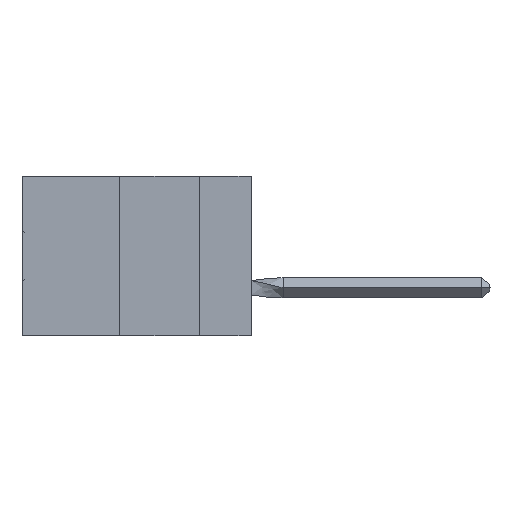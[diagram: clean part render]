
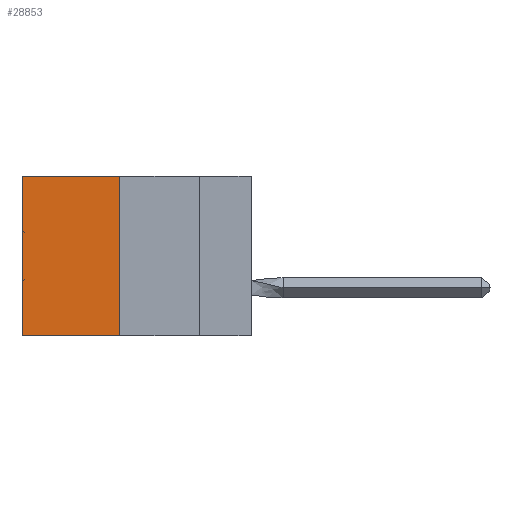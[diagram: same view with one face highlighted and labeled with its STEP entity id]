
A CAD part, left-side view. The second image highlights one B-rep face of the part: STEP entity #28853.
In plain terms, the highlighted planar face has unit normal (-1, 0, 0).
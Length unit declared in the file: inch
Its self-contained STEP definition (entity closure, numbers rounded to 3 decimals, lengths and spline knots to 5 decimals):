
#2161 = CARTESIAN_POINT ( 'NONE',  ( 0.305, 0.413, 0. ) ) ;
#4293 = DIRECTION ( 'NONE',  ( 0., 0., -1. ) ) ;
#4433 = EDGE_LOOP ( 'NONE', ( #32694, #45407, #19764, #10352 ) ) ;
#4659 = CARTESIAN_POINT ( 'NONE',  ( 0.305, 0.72, -0.5 ) ) ;
#6566 = CARTESIAN_POINT ( 'NONE',  ( 0.305, 0.72, -0.5 ) ) ;
#8928 = DIRECTION ( 'NONE',  ( 0., 1., 0. ) ) ;
#9058 = CARTESIAN_POINT ( 'NONE',  ( 0.305, 0.72, 0. ) ) ;
#9150 = EDGE_CURVE ( 'NONE', #37162, #15624, #11273, .T. ) ;
#10037 = DIRECTION ( 'NONE',  ( 0., 1., 0. ) ) ;
#10352 = ORIENTED_EDGE ( 'NONE', *, *, #23976, .T. ) ;
#10366 = CARTESIAN_POINT ( 'NONE',  ( 0.305, 0.413, -0.5 ) ) ;
#11273 = LINE ( 'NONE', #4659, #19214 ) ;
#13150 = LINE ( 'NONE', #2161, #17441 ) ;
#15624 = VERTEX_POINT ( 'NONE', #6566 ) ;
#16854 = AXIS2_PLACEMENT_3D ( 'NONE', #23687, #27618, #4293 ) ;
#17441 = VECTOR ( 'NONE', #10037, 39.37008 ) ;
#17703 = EDGE_CURVE ( 'NONE', #46464, #30161, #50212, .T. ) ;
#19214 = VECTOR ( 'NONE', #24394, 39.37008 ) ;
#19764 = ORIENTED_EDGE ( 'NONE', *, *, #17703, .F. ) ;
#20530 = VECTOR ( 'NONE', #8928, 39.37008 ) ;
#20861 = VECTOR ( 'NONE', #29987, 39.37008 ) ;
#21524 = FACE_OUTER_BOUND ( 'NONE', #4433, .T. ) ;
#23687 = CARTESIAN_POINT ( 'NONE',  ( 0.305, 0.413, -0.5 ) ) ;
#23976 = EDGE_CURVE ( 'NONE', #46464, #37162, #13150, .T. ) ;
#24394 = DIRECTION ( 'NONE',  ( 0., 0., -1. ) ) ;
#27618 = DIRECTION ( 'NONE',  ( 1., 0., 0. ) ) ;
#28853 = ADVANCED_FACE ( 'NONE', ( #21524 ), #47112, .F. ) ;
#29987 = DIRECTION ( 'NONE',  ( 0., 0., -1. ) ) ;
#30161 = VERTEX_POINT ( 'NONE', #38555 ) ;
#31324 = CARTESIAN_POINT ( 'NONE',  ( 0.305, 0.413, 0. ) ) ;
#31478 = LINE ( 'NONE', #43950, #20530 ) ;
#32694 = ORIENTED_EDGE ( 'NONE', *, *, #9150, .T. ) ;
#33674 = EDGE_CURVE ( 'NONE', #30161, #15624, #31478, .T. ) ;
#37162 = VERTEX_POINT ( 'NONE', #9058 ) ;
#38555 = CARTESIAN_POINT ( 'NONE',  ( 0.305, 0.413, -0.5 ) ) ;
#43950 = CARTESIAN_POINT ( 'NONE',  ( 0.305, 0.413, -0.5 ) ) ;
#45407 = ORIENTED_EDGE ( 'NONE', *, *, #33674, .F. ) ;
#46464 = VERTEX_POINT ( 'NONE', #31324 ) ;
#47112 = PLANE ( 'NONE',  #16854 ) ;
#50212 = LINE ( 'NONE', #10366, #20861 ) ;
